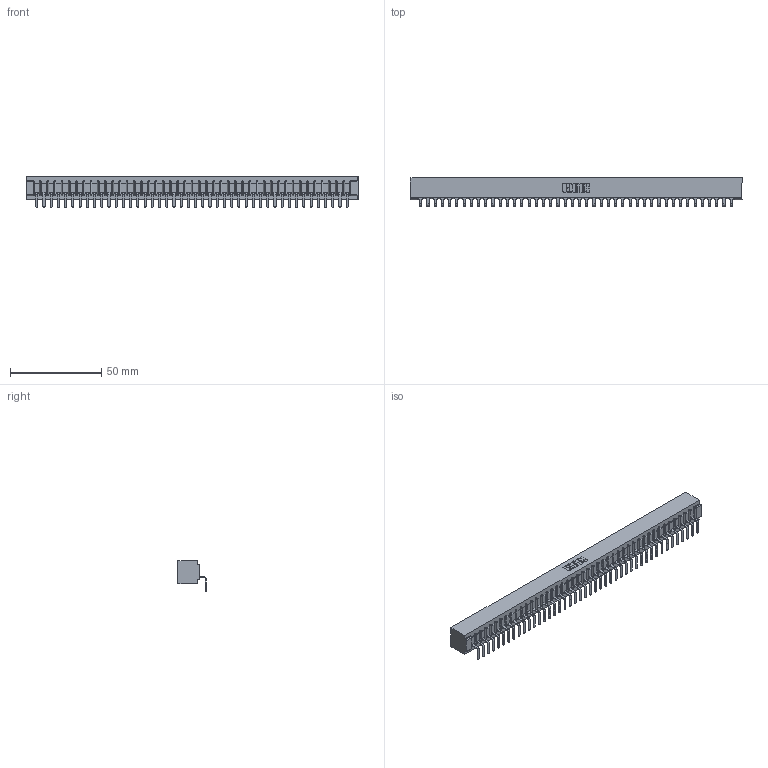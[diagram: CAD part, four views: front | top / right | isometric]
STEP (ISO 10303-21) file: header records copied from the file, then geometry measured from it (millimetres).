
FILE_DESCRIPTION (( 'STEP AP203' ), '1' );
FILE_NAME ('307-044-559-101.STEP', '2019-09-05T17:30:15', ( '' ), ( '' ), 'SwSTEP 2.0', 'SolidWorks 2016', '' );
FILE_SCHEMA (( 'CONFIG_CONTROL_DESIGN' ));
Length unit declared in the file: inch
Products named in the file (3): 307-290-001_558 559 - 1 (Single); 307-044-559-101; 307 Part_No Mounting Lugs
Assembly tree (45 placements, depth 2):
  307-044-559-101
    307 Part_No Mounting Lugs
    307-290-001_558 559 - 1 (Single)  x44
Bounding box: 182.22 x 15.46 x 16.8 mm (x, y, z)
Volume: 19491.1 mm3; surface area: 21122.3 mm2
Topology: 45 solids, 45 shells, 2795 faces, 7955 edges, 5122 vertices
Faces by surface type: plane 1782, cylinder 923, sphere 90
Entity records: 37300 total; most frequent: CARTESIAN_POINT 6284, ORIENTED_EDGE 6270, DIRECTION 6109, EDGE_CURVE 3135, LINE 2407, VECTOR 2407, VERTEX_POINT 2026, AXIS2_PLACEMENT_3D 1851
